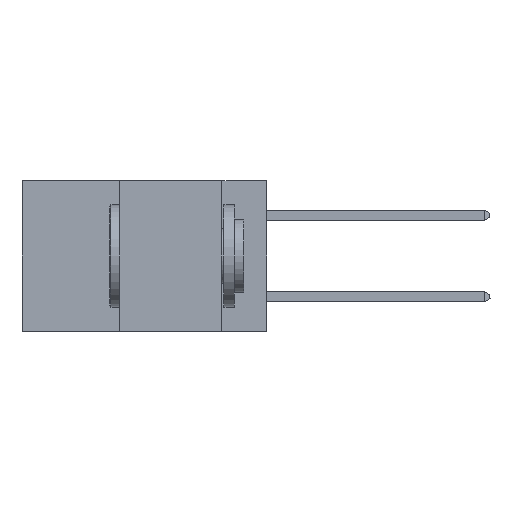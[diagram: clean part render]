
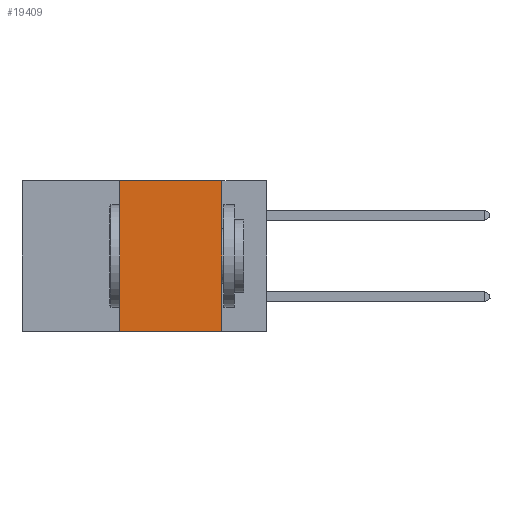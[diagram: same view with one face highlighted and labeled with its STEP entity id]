
A CAD part, left-side view. The second image highlights one B-rep face of the part: STEP entity #19409.
In plain terms, the highlighted planar face has unit normal (-1, 0, 0).
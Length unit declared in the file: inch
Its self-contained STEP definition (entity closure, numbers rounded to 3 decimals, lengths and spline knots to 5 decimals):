
#1061 = AXIS2_PLACEMENT_3D ( 'NONE', #9430, #34114, #9312 ) ;
#1172 = CARTESIAN_POINT ( 'NONE',  ( 0., 0.11, -0.37 ) ) ;
#2779 = LINE ( 'NONE', #26872, #7522 ) ;
#3600 = CARTESIAN_POINT ( 'NONE',  ( 0., 0.11, 0. ) ) ;
#5244 = VERTEX_POINT ( 'NONE', #16351 ) ;
#6048 = VERTEX_POINT ( 'NONE', #3600 ) ;
#6766 = CARTESIAN_POINT ( 'NONE',  ( 0., 0.36, 0. ) ) ;
#6792 = EDGE_CURVE ( 'NONE', #6048, #23523, #2779, .T. ) ;
#7320 = EDGE_CURVE ( 'NONE', #5244, #9422, #16540, .T. ) ;
#7522 = VECTOR ( 'NONE', #13105, 39.37008 ) ;
#9195 = VECTOR ( 'NONE', #23194, 39.37008 ) ;
#9312 = DIRECTION ( 'NONE',  ( 0., 0., -1. ) ) ;
#9422 = VERTEX_POINT ( 'NONE', #24542 ) ;
#9430 = CARTESIAN_POINT ( 'NONE',  ( 0., 0.6, 0. ) ) ;
#10934 = LINE ( 'NONE', #11169, #20930 ) ;
#11169 = CARTESIAN_POINT ( 'NONE',  ( 0., 0.6, -0.37 ) ) ;
#12266 = VECTOR ( 'NONE', #33446, 39.37008 ) ;
#12389 = ORIENTED_EDGE ( 'NONE', *, *, #22092, .F. ) ;
#13009 = EDGE_CURVE ( 'NONE', #5244, #23523, #10934, .T. ) ;
#13105 = DIRECTION ( 'NONE',  ( 0., 0., -1. ) ) ;
#14446 = LINE ( 'NONE', #22749, #12266 ) ;
#16351 = CARTESIAN_POINT ( 'NONE',  ( 0., 0.36, -0.37 ) ) ;
#16540 = LINE ( 'NONE', #6766, #9195 ) ;
#19409 = ADVANCED_FACE ( 'NONE', ( #28121 ), #25819, .F. ) ;
#19535 = DIRECTION ( 'NONE',  ( 0., -1., 0. ) ) ;
#20930 = VECTOR ( 'NONE', #19535, 39.37008 ) ;
#22092 = EDGE_CURVE ( 'NONE', #9422, #6048, #14446, .T. ) ;
#22749 = CARTESIAN_POINT ( 'NONE',  ( 0., 0.6, 0. ) ) ;
#23194 = DIRECTION ( 'NONE',  ( 0., 0., 1. ) ) ;
#23523 = VERTEX_POINT ( 'NONE', #1172 ) ;
#24542 = CARTESIAN_POINT ( 'NONE',  ( 0., 0.36, 0. ) ) ;
#25246 = ORIENTED_EDGE ( 'NONE', *, *, #7320, .F. ) ;
#25819 = PLANE ( 'NONE',  #1061 ) ;
#26872 = CARTESIAN_POINT ( 'NONE',  ( 0., 0.11, 0. ) ) ;
#26922 = ORIENTED_EDGE ( 'NONE', *, *, #6792, .F. ) ;
#28121 = FACE_OUTER_BOUND ( 'NONE', #34473, .T. ) ;
#30148 = ORIENTED_EDGE ( 'NONE', *, *, #13009, .T. ) ;
#33446 = DIRECTION ( 'NONE',  ( 0., -1., 0. ) ) ;
#34114 = DIRECTION ( 'NONE',  ( 1., 0., 0. ) ) ;
#34473 = EDGE_LOOP ( 'NONE', ( #26922, #12389, #25246, #30148 ) ) ;
